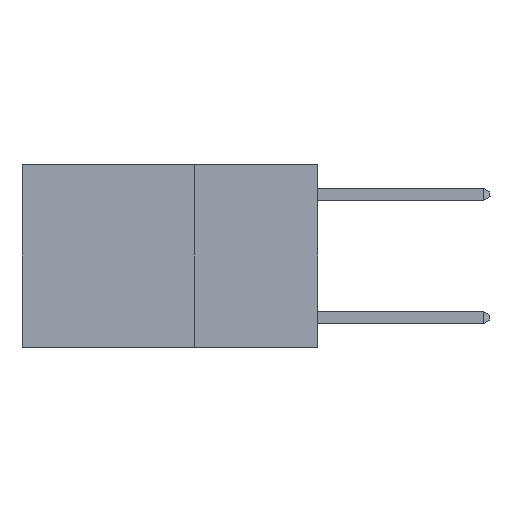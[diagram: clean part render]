
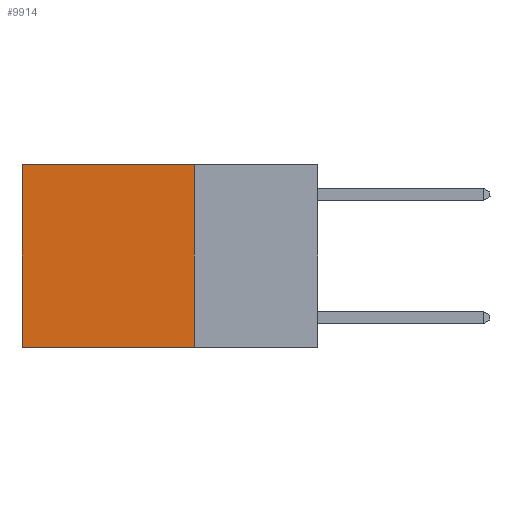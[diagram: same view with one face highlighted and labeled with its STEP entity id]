
A CAD part, left-side view. The second image highlights one B-rep face of the part: STEP entity #9914.
In plain terms, the highlighted planar face has unit normal (-1, 0, 0).
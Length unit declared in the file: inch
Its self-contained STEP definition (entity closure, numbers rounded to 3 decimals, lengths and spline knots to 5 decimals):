
#495 = EDGE_CURVE ( 'NONE', #10162, #7738, #8195, .T. ) ;
#612 = PLANE ( 'NONE',  #5089 ) ;
#1295 = DIRECTION ( 'NONE',  ( 0., 0., -1. ) ) ;
#1408 = DIRECTION ( 'NONE',  ( 1., 0., 0. ) ) ;
#1446 = LINE ( 'NONE', #4980, #6073 ) ;
#1480 = CARTESIAN_POINT ( 'NONE',  ( 0.2625, 0.25, -0.37 ) ) ;
#1810 = ORIENTED_EDGE ( 'NONE', *, *, #495, .F. ) ;
#2128 = DIRECTION ( 'NONE',  ( 0., 0., -1. ) ) ;
#2327 = EDGE_LOOP ( 'NONE', ( #10885, #3203, #1810, #3452 ) ) ;
#2428 = DIRECTION ( 'NONE',  ( 0., 0., -1. ) ) ;
#2782 = CARTESIAN_POINT ( 'NONE',  ( 0.2625, 0.25, -0.37 ) ) ;
#2896 = DIRECTION ( 'NONE',  ( 0., 1., 0. ) ) ;
#3203 = ORIENTED_EDGE ( 'NONE', *, *, #3651, .F. ) ;
#3452 = ORIENTED_EDGE ( 'NONE', *, *, #3665, .T. ) ;
#3651 = EDGE_CURVE ( 'NONE', #7738, #8792, #8008, .T. ) ;
#3665 = EDGE_CURVE ( 'NONE', #10162, #3811, #7892, .T. ) ;
#3811 = VERTEX_POINT ( 'NONE', #9967 ) ;
#4845 = FACE_OUTER_BOUND ( 'NONE', #2327, .T. ) ;
#4980 = CARTESIAN_POINT ( 'NONE',  ( 0.2625, 0.6, 0. ) ) ;
#5089 = AXIS2_PLACEMENT_3D ( 'NONE', #10809, #1408, #2128 ) ;
#5230 = CARTESIAN_POINT ( 'NONE',  ( 0.2625, 0.25, 0. ) ) ;
#6073 = VECTOR ( 'NONE', #2428, 39.37008 ) ;
#6279 = CARTESIAN_POINT ( 'NONE',  ( 0.2625, 0.25, 0. ) ) ;
#7162 = DIRECTION ( 'NONE',  ( 0., 1., 0. ) ) ;
#7354 = EDGE_CURVE ( 'NONE', #3811, #8792, #1446, .T. ) ;
#7458 = VECTOR ( 'NONE', #7162, 39.37008 ) ;
#7738 = VERTEX_POINT ( 'NONE', #1480 ) ;
#7892 = LINE ( 'NONE', #6279, #7458 ) ;
#8008 = LINE ( 'NONE', #2782, #8182 ) ;
#8182 = VECTOR ( 'NONE', #2896, 39.37008 ) ;
#8195 = LINE ( 'NONE', #9718, #9168 ) ;
#8792 = VERTEX_POINT ( 'NONE', #9378 ) ;
#9168 = VECTOR ( 'NONE', #1295, 39.37008 ) ;
#9378 = CARTESIAN_POINT ( 'NONE',  ( 0.2625, 0.6, -0.37 ) ) ;
#9718 = CARTESIAN_POINT ( 'NONE',  ( 0.2625, 0.25, 0. ) ) ;
#9914 = ADVANCED_FACE ( 'NONE', ( #4845 ), #612, .F. ) ;
#9967 = CARTESIAN_POINT ( 'NONE',  ( 0.2625, 0.6, 0. ) ) ;
#10162 = VERTEX_POINT ( 'NONE', #5230 ) ;
#10809 = CARTESIAN_POINT ( 'NONE',  ( 0.2625, 0.25, 0. ) ) ;
#10885 = ORIENTED_EDGE ( 'NONE', *, *, #7354, .T. ) ;
